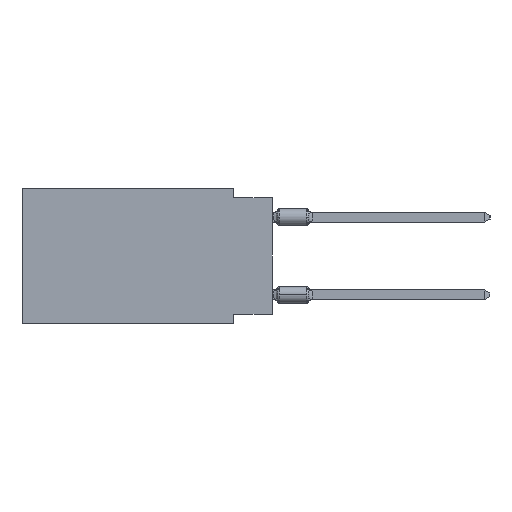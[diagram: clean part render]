
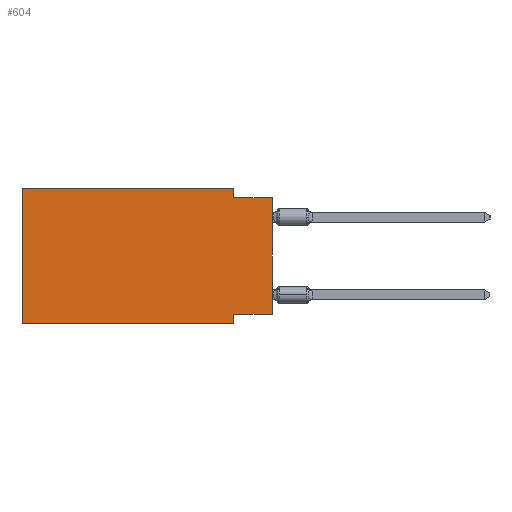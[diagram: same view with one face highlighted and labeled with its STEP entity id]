
A CAD part, left-side view. The second image highlights one B-rep face of the part: STEP entity #604.
In plain terms, the highlighted planar face has unit normal (-1, 0, 0).
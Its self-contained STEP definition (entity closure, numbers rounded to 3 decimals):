
#253 = EDGE_CURVE ( 'NONE', #20111, #35591, #6791, .T. ) ;
#604 = ADVANCED_FACE ( 'NONE', ( #42084 ), #2233, .F. ) ;
#885 = LINE ( 'NONE', #12868, #40412 ) ;
#2233 = PLANE ( 'NONE',  #14512 ) ;
#3349 = CARTESIAN_POINT ( 'NONE',  ( 0., 16.383, 0. ) ) ;
#3966 = VERTEX_POINT ( 'NONE', #15498 ) ;
#4595 = DIRECTION ( 'NONE',  ( 0., 0., -1. ) ) ;
#5171 = LINE ( 'NONE', #35939, #18428 ) ;
#5238 = CARTESIAN_POINT ( 'NONE',  ( 0., 2.54, -8.255 ) ) ;
#6281 = DIRECTION ( 'NONE',  ( 0., -1., 0. ) ) ;
#6544 = CARTESIAN_POINT ( 'NONE',  ( 0., 2.54, -0.635 ) ) ;
#6791 = LINE ( 'NONE', #54883, #49938 ) ;
#7127 = LINE ( 'NONE', #54944, #48869 ) ;
#7586 = VECTOR ( 'NONE', #27069, 1000. ) ;
#7636 = DIRECTION ( 'NONE',  ( 0., -1., 0. ) ) ;
#8745 = CARTESIAN_POINT ( 'NONE',  ( 0., 16.383, 0. ) ) ;
#9733 = EDGE_CURVE ( 'NONE', #17037, #35870, #7127, .T. ) ;
#10186 = LINE ( 'NONE', #48910, #22249 ) ;
#12754 = LINE ( 'NONE', #8745, #15430 ) ;
#12868 = CARTESIAN_POINT ( 'NONE',  ( 0., 2.54, 0. ) ) ;
#14460 = ORIENTED_EDGE ( 'NONE', *, *, #253, .T. ) ;
#14512 = AXIS2_PLACEMENT_3D ( 'NONE', #3349, #54884, #37538 ) ;
#15430 = VECTOR ( 'NONE', #30124, 1000. ) ;
#15498 = CARTESIAN_POINT ( 'NONE',  ( 0., 2.54, 0. ) ) ;
#17037 = VERTEX_POINT ( 'NONE', #6544 ) ;
#18428 = VECTOR ( 'NONE', #31390, 1000. ) ;
#20111 = VERTEX_POINT ( 'NONE', #23353 ) ;
#20822 = ORIENTED_EDGE ( 'NONE', *, *, #9733, .F. ) ;
#20948 = ORIENTED_EDGE ( 'NONE', *, *, #47323, .F. ) ;
#22249 = VECTOR ( 'NONE', #48072, 1000. ) ;
#22676 = VECTOR ( 'NONE', #7636, 1000. ) ;
#23353 = CARTESIAN_POINT ( 'NONE',  ( 0., 16.383, -8.89 ) ) ;
#23970 = ORIENTED_EDGE ( 'NONE', *, *, #43093, .F. ) ;
#25078 = ORIENTED_EDGE ( 'NONE', *, *, #30849, .F. ) ;
#27069 = DIRECTION ( 'NONE',  ( 0., 1., 0. ) ) ;
#30124 = DIRECTION ( 'NONE',  ( 0., 0., 1. ) ) ;
#30527 = ORIENTED_EDGE ( 'NONE', *, *, #38734, .T. ) ;
#30849 = EDGE_CURVE ( 'NONE', #38591, #49073, #39580, .T. ) ;
#31390 = DIRECTION ( 'NONE',  ( 0., 0., -1. ) ) ;
#33193 = ORIENTED_EDGE ( 'NONE', *, *, #47334, .F. ) ;
#34665 = EDGE_CURVE ( 'NONE', #49073, #35591, #5171, .T. ) ;
#35591 = VERTEX_POINT ( 'NONE', #41428 ) ;
#35870 = VERTEX_POINT ( 'NONE', #39656 ) ;
#35939 = CARTESIAN_POINT ( 'NONE',  ( 0., 2.54, -8.89 ) ) ;
#37538 = DIRECTION ( 'NONE',  ( 0., 0., -1. ) ) ;
#38379 = LINE ( 'NONE', #51736, #22676 ) ;
#38591 = VERTEX_POINT ( 'NONE', #47793 ) ;
#38734 = EDGE_CURVE ( 'NONE', #38591, #35870, #10186, .T. ) ;
#39580 = LINE ( 'NONE', #52641, #7586 ) ;
#39656 = CARTESIAN_POINT ( 'NONE',  ( 0., 0., -0.635 ) ) ;
#40412 = VECTOR ( 'NONE', #4595, 1000. ) ;
#41428 = CARTESIAN_POINT ( 'NONE',  ( 0., 2.54, -8.89 ) ) ;
#42084 = FACE_OUTER_BOUND ( 'NONE', #47558, .T. ) ;
#43093 = EDGE_CURVE ( 'NONE', #3966, #17037, #885, .T. ) ;
#47323 = EDGE_CURVE ( 'NONE', #20111, #54104, #12754, .T. ) ;
#47334 = EDGE_CURVE ( 'NONE', #54104, #3966, #38379, .T. ) ;
#47558 = EDGE_LOOP ( 'NONE', ( #30527, #20822, #23970, #33193, #20948, #14460, #48440, #25078 ) ) ;
#47793 = CARTESIAN_POINT ( 'NONE',  ( 0., 0., -8.255 ) ) ;
#48072 = DIRECTION ( 'NONE',  ( 0., 0., 1. ) ) ;
#48440 = ORIENTED_EDGE ( 'NONE', *, *, #34665, .F. ) ;
#48869 = VECTOR ( 'NONE', #6281, 1000. ) ;
#48910 = CARTESIAN_POINT ( 'NONE',  ( 0., 0., 0. ) ) ;
#49073 = VERTEX_POINT ( 'NONE', #5238 ) ;
#49938 = VECTOR ( 'NONE', #54043, 1000. ) ;
#51736 = CARTESIAN_POINT ( 'NONE',  ( 0., 16.383, 0. ) ) ;
#52641 = CARTESIAN_POINT ( 'NONE',  ( 0., 0., -8.255 ) ) ;
#53589 = CARTESIAN_POINT ( 'NONE',  ( 0., 16.383, 0. ) ) ;
#54043 = DIRECTION ( 'NONE',  ( 0., -1., 0. ) ) ;
#54104 = VERTEX_POINT ( 'NONE', #53589 ) ;
#54883 = CARTESIAN_POINT ( 'NONE',  ( 0., 16.383, -8.89 ) ) ;
#54884 = DIRECTION ( 'NONE',  ( 1., 0., 0. ) ) ;
#54944 = CARTESIAN_POINT ( 'NONE',  ( 0., 0., -0.635 ) ) ;
